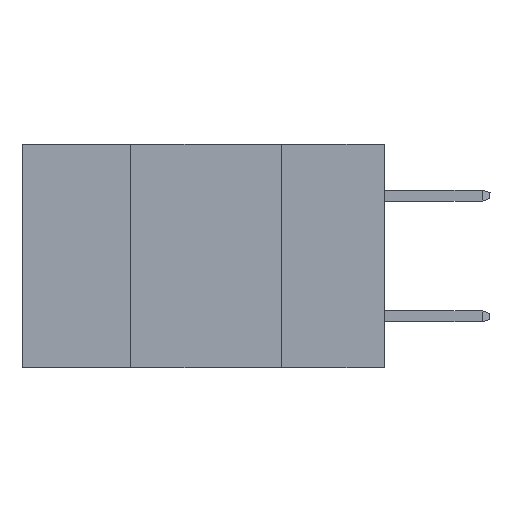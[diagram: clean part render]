
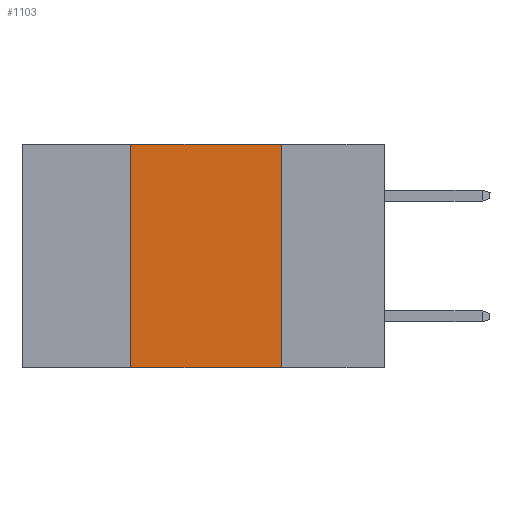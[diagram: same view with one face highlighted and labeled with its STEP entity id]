
A CAD part, left-side view. The second image highlights one B-rep face of the part: STEP entity #1103.
In plain terms, the highlighted planar face has unit normal (-1, 0, 0).
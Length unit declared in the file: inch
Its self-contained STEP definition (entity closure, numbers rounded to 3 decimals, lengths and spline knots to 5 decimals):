
#121 = ORIENTED_EDGE ( 'NONE', *, *, #12890, .F. ) ;
#999 = CARTESIAN_POINT ( 'NONE',  ( 0., 0.17, 0. ) ) ;
#1103 = ADVANCED_FACE ( 'NONE', ( #24118 ), #4777, .F. ) ;
#1922 = CARTESIAN_POINT ( 'NONE',  ( 0., 0.6, -0.37 ) ) ;
#2873 = VERTEX_POINT ( 'NONE', #24413 ) ;
#3232 = DIRECTION ( 'NONE',  ( 0., 0., -1. ) ) ;
#3624 = CARTESIAN_POINT ( 'NONE',  ( 0., 0.6, 0. ) ) ;
#4612 = DIRECTION ( 'NONE',  ( 0., -1., 0. ) ) ;
#4777 = PLANE ( 'NONE',  #11339 ) ;
#7536 = ORIENTED_EDGE ( 'NONE', *, *, #22085, .F. ) ;
#9066 = LINE ( 'NONE', #1922, #22685 ) ;
#9516 = VERTEX_POINT ( 'NONE', #19030 ) ;
#11079 = CARTESIAN_POINT ( 'NONE',  ( 0., 0.6, 0. ) ) ;
#11249 = DIRECTION ( 'NONE',  ( 1., 0., 0. ) ) ;
#11339 = AXIS2_PLACEMENT_3D ( 'NONE', #11079, #11249, #15150 ) ;
#11471 = EDGE_CURVE ( 'NONE', #25379, #20998, #9066, .T. ) ;
#11651 = VECTOR ( 'NONE', #12211, 39.37008 ) ;
#12097 = VECTOR ( 'NONE', #19636, 39.37008 ) ;
#12211 = DIRECTION ( 'NONE',  ( 0., 0., 1. ) ) ;
#12890 = EDGE_CURVE ( 'NONE', #2873, #20998, #21948, .T. ) ;
#15150 = DIRECTION ( 'NONE',  ( 0., 0., -1. ) ) ;
#17960 = CARTESIAN_POINT ( 'NONE',  ( 0., 0.42, -0.37 ) ) ;
#18339 = EDGE_CURVE ( 'NONE', #9516, #2873, #18742, .T. ) ;
#18742 = LINE ( 'NONE', #3624, #12097 ) ;
#19030 = CARTESIAN_POINT ( 'NONE',  ( 0., 0.42, 0. ) ) ;
#19146 = VECTOR ( 'NONE', #3232, 39.37008 ) ;
#19636 = DIRECTION ( 'NONE',  ( 0., -1., 0. ) ) ;
#20096 = ORIENTED_EDGE ( 'NONE', *, *, #18339, .F. ) ;
#20998 = VERTEX_POINT ( 'NONE', #21172 ) ;
#21172 = CARTESIAN_POINT ( 'NONE',  ( 0., 0.17, -0.37 ) ) ;
#21948 = LINE ( 'NONE', #999, #19146 ) ;
#22053 = ORIENTED_EDGE ( 'NONE', *, *, #11471, .T. ) ;
#22085 = EDGE_CURVE ( 'NONE', #25379, #9516, #25859, .T. ) ;
#22617 = CARTESIAN_POINT ( 'NONE',  ( 0., 0.42, 0. ) ) ;
#22685 = VECTOR ( 'NONE', #4612, 39.37008 ) ;
#24118 = FACE_OUTER_BOUND ( 'NONE', #25481, .T. ) ;
#24413 = CARTESIAN_POINT ( 'NONE',  ( 0., 0.17, 0. ) ) ;
#25379 = VERTEX_POINT ( 'NONE', #17960 ) ;
#25481 = EDGE_LOOP ( 'NONE', ( #121, #20096, #7536, #22053 ) ) ;
#25859 = LINE ( 'NONE', #22617, #11651 ) ;
